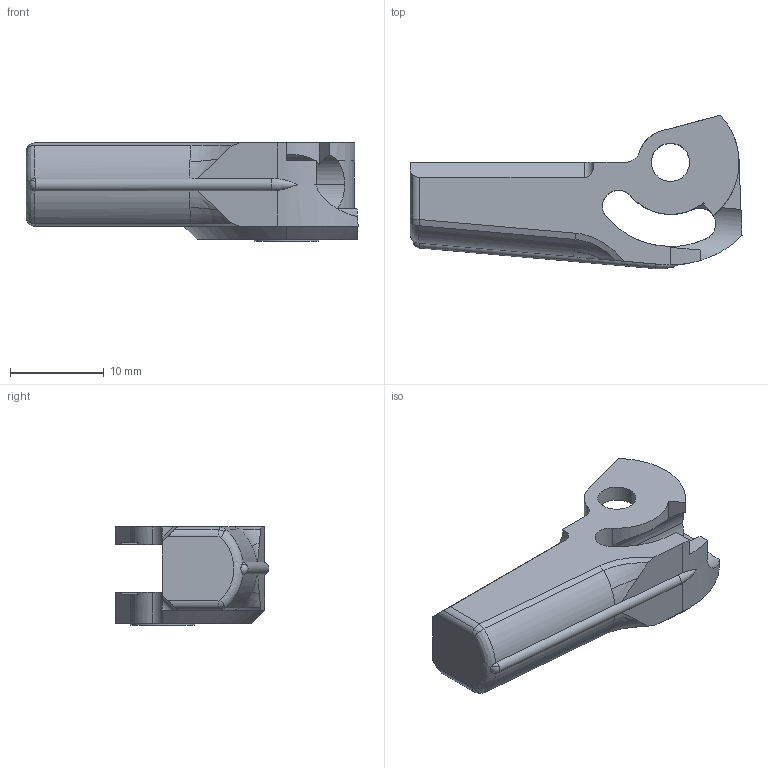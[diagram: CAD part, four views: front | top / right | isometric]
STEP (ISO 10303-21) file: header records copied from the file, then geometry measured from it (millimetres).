
FILE_DESCRIPTION (( 'STEP AP214' ), '1' );
FILE_NAME ('Hammer.step', '2014-07-30T19:46:01', ( 'WarFairy' ), ( '' ), 'SwSTEP 2.0', 'SolidWorks 2013', '' );
FILE_SCHEMA (( 'AUTOMOTIVE_DESIGN' ));
Length unit declared in the file: millimetre
Products named in the file (1): Hammer
Bounding box: 35.51 x 16.43 x 10.5 mm (x, y, z)
Volume: 1680.6 mm3; surface area: 2295.5 mm2
Topology: 1 solids, 1 shells, 85 faces, 252 edges, 166 vertices
Faces by surface type: cylinder 40, plane 33, torus 5, bspline 3, sphere 2, cone 2
Entity records: 3353 total; most frequent: CARTESIAN_POINT 1159, ORIENTED_EDGE 496, DIRECTION 410, EDGE_CURVE 248, VERTEX_POINT 164, AXIS2_PLACEMENT_3D 144, LINE 122, VECTOR 122
